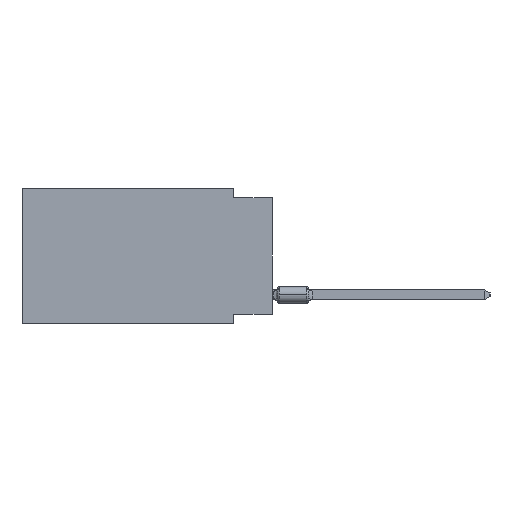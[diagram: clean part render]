
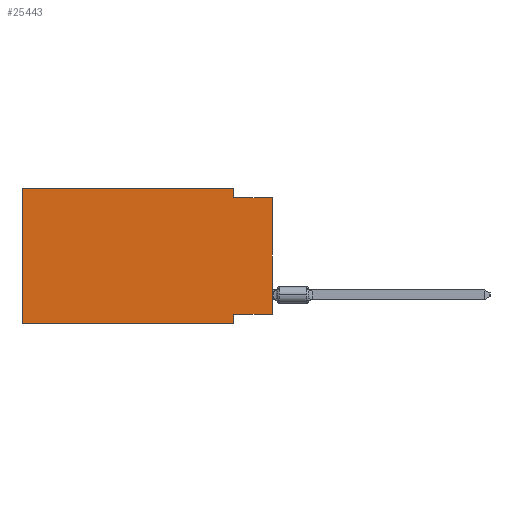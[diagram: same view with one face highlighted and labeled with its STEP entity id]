
A CAD part, left-side view. The second image highlights one B-rep face of the part: STEP entity #25443.
In plain terms, the highlighted planar face has unit normal (-1, 0, 0).
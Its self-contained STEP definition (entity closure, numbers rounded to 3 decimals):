
#114 = ORIENTED_EDGE ( 'NONE', *, *, #12732, .F. ) ;
#279 = DIRECTION ( 'NONE',  ( 0., -1., 0. ) ) ;
#359 = VERTEX_POINT ( 'NONE', #568 ) ;
#568 = CARTESIAN_POINT ( 'NONE',  ( 0., 16.383, -8.89 ) ) ;
#2121 = DIRECTION ( 'NONE',  ( 0., 0., 1. ) ) ;
#3538 = CARTESIAN_POINT ( 'NONE',  ( 0., 0., -0.635 ) ) ;
#4005 = ORIENTED_EDGE ( 'NONE', *, *, #51577, .F. ) ;
#4865 = DIRECTION ( 'NONE',  ( 0., 0., -1. ) ) ;
#5841 = CARTESIAN_POINT ( 'NONE',  ( 0., 16.383, 0. ) ) ;
#5931 = ORIENTED_EDGE ( 'NONE', *, *, #8891, .T. ) ;
#7966 = VERTEX_POINT ( 'NONE', #5841 ) ;
#8891 = EDGE_CURVE ( 'NONE', #359, #60574, #48920, .T. ) ;
#8940 = VECTOR ( 'NONE', #65703, 1000. ) ;
#8987 = DIRECTION ( 'NONE',  ( 0., 0., -1. ) ) ;
#9125 = ORIENTED_EDGE ( 'NONE', *, *, #60482, .T. ) ;
#10164 = VECTOR ( 'NONE', #8987, 1000. ) ;
#10803 = EDGE_CURVE ( 'NONE', #359, #7966, #37635, .T. ) ;
#10971 = VECTOR ( 'NONE', #2121, 1000. ) ;
#11747 = LINE ( 'NONE', #54377, #30943 ) ;
#12485 = AXIS2_PLACEMENT_3D ( 'NONE', #30398, #52426, #4865 ) ;
#12630 = CARTESIAN_POINT ( 'NONE',  ( 0., 2.54, -8.89 ) ) ;
#12732 = EDGE_CURVE ( 'NONE', #39285, #60574, #20124, .T. ) ;
#12903 = EDGE_CURVE ( 'NONE', #7966, #49639, #38229, .T. ) ;
#16106 = VECTOR ( 'NONE', #279, 1000. ) ;
#19013 = VECTOR ( 'NONE', #65254, 1000. ) ;
#19458 = VERTEX_POINT ( 'NONE', #25360 ) ;
#20124 = LINE ( 'NONE', #26041, #61235 ) ;
#22853 = DIRECTION ( 'NONE',  ( 0., -1., 0. ) ) ;
#23036 = CARTESIAN_POINT ( 'NONE',  ( 0., 16.383, -8.89 ) ) ;
#25040 = LINE ( 'NONE', #30279, #10164 ) ;
#25360 = CARTESIAN_POINT ( 'NONE',  ( 0., 0., -8.255 ) ) ;
#25443 = ADVANCED_FACE ( 'NONE', ( #47517 ), #52768, .F. ) ;
#26041 = CARTESIAN_POINT ( 'NONE',  ( 0., 2.54, -8.89 ) ) ;
#27126 = DIRECTION ( 'NONE',  ( 0., 1., 0. ) ) ;
#29628 = VERTEX_POINT ( 'NONE', #36416 ) ;
#30010 = ORIENTED_EDGE ( 'NONE', *, *, #10803, .F. ) ;
#30279 = CARTESIAN_POINT ( 'NONE',  ( 0., 2.54, 0. ) ) ;
#30398 = CARTESIAN_POINT ( 'NONE',  ( 0., 16.383, 0. ) ) ;
#30943 = VECTOR ( 'NONE', #27126, 1000. ) ;
#31263 = EDGE_CURVE ( 'NONE', #19458, #39285, #11747, .T. ) ;
#32712 = ORIENTED_EDGE ( 'NONE', *, *, #44121, .F. ) ;
#36416 = CARTESIAN_POINT ( 'NONE',  ( 0., 2.54, -0.635 ) ) ;
#37635 = LINE ( 'NONE', #43917, #19013 ) ;
#38229 = LINE ( 'NONE', #59917, #55643 ) ;
#39285 = VERTEX_POINT ( 'NONE', #61058 ) ;
#43917 = CARTESIAN_POINT ( 'NONE',  ( 0., 16.383, 0. ) ) ;
#44121 = EDGE_CURVE ( 'NONE', #49639, #29628, #25040, .T. ) ;
#44414 = CARTESIAN_POINT ( 'NONE',  ( 0., 0., 0. ) ) ;
#44964 = VERTEX_POINT ( 'NONE', #3538 ) ;
#45153 = EDGE_LOOP ( 'NONE', ( #9125, #4005, #32712, #58883, #30010, #5931, #114, #52698 ) ) ;
#47139 = LINE ( 'NONE', #68488, #16106 ) ;
#47358 = DIRECTION ( 'NONE',  ( 0., 0., -1. ) ) ;
#47517 = FACE_OUTER_BOUND ( 'NONE', #45153, .T. ) ;
#48284 = LINE ( 'NONE', #44414, #10971 ) ;
#48920 = LINE ( 'NONE', #23036, #8940 ) ;
#49639 = VERTEX_POINT ( 'NONE', #61925 ) ;
#51577 = EDGE_CURVE ( 'NONE', #29628, #44964, #47139, .T. ) ;
#52426 = DIRECTION ( 'NONE',  ( 1., 0., 0. ) ) ;
#52698 = ORIENTED_EDGE ( 'NONE', *, *, #31263, .F. ) ;
#52768 = PLANE ( 'NONE',  #12485 ) ;
#54377 = CARTESIAN_POINT ( 'NONE',  ( 0., 0., -8.255 ) ) ;
#55643 = VECTOR ( 'NONE', #22853, 1000. ) ;
#58883 = ORIENTED_EDGE ( 'NONE', *, *, #12903, .F. ) ;
#59917 = CARTESIAN_POINT ( 'NONE',  ( 0., 16.383, 0. ) ) ;
#60482 = EDGE_CURVE ( 'NONE', #19458, #44964, #48284, .T. ) ;
#60574 = VERTEX_POINT ( 'NONE', #12630 ) ;
#61058 = CARTESIAN_POINT ( 'NONE',  ( 0., 2.54, -8.255 ) ) ;
#61235 = VECTOR ( 'NONE', #47358, 1000. ) ;
#61925 = CARTESIAN_POINT ( 'NONE',  ( 0., 2.54, 0. ) ) ;
#65254 = DIRECTION ( 'NONE',  ( 0., 0., 1. ) ) ;
#65703 = DIRECTION ( 'NONE',  ( 0., -1., 0. ) ) ;
#68488 = CARTESIAN_POINT ( 'NONE',  ( 0., 0., -0.635 ) ) ;
